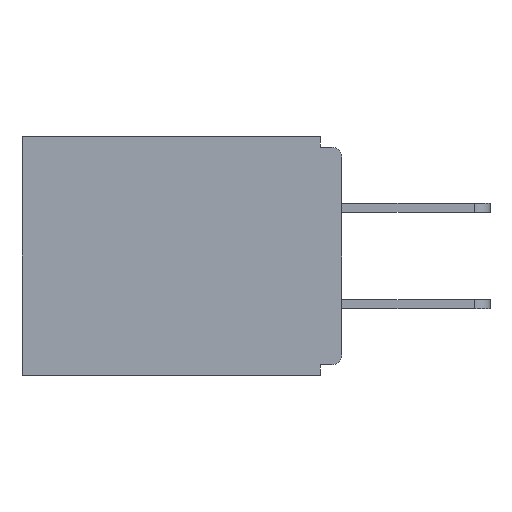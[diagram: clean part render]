
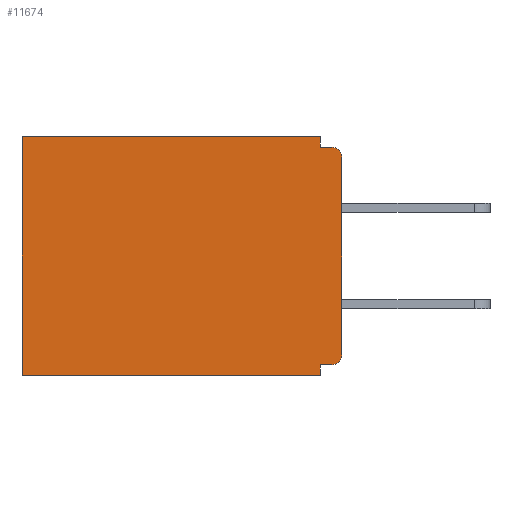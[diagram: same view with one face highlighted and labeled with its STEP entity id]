
A CAD part, left-side view. The second image highlights one B-rep face of the part: STEP entity #11674.
In plain terms, the highlighted planar face has unit normal (-1, 0, 0).
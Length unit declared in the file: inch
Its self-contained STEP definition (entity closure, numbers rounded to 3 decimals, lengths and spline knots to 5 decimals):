
#292 = CARTESIAN_POINT ( 'NONE',  ( 0.298, 0.46, 0. ) ) ;
#1501 = CARTESIAN_POINT ( 'NONE',  ( 0.298, 0.46, -0.343 ) ) ;
#1560 = EDGE_CURVE ( 'NONE', #3547, #20844, #1726, .T. ) ;
#1709 = ORIENTED_EDGE ( 'NONE', *, *, #22914, .T. ) ;
#1726 = LINE ( 'NONE', #8115, #23802 ) ;
#1898 = EDGE_CURVE ( 'NONE', #21449, #11627, #26825, .T. ) ;
#2125 = EDGE_CURVE ( 'NONE', #12334, #6554, #13022, .T. ) ;
#2686 = EDGE_CURVE ( 'NONE', #12334, #3741, #8973, .T. ) ;
#2949 = DIRECTION ( 'NONE',  ( -1., 0., 0. ) ) ;
#3547 = VERTEX_POINT ( 'NONE', #9557 ) ;
#3594 = VECTOR ( 'NONE', #25266, 39.37008 ) ;
#3741 = VERTEX_POINT ( 'NONE', #12720 ) ;
#3879 = CARTESIAN_POINT ( 'NONE',  ( 0.298, 0., -0.328 ) ) ;
#4318 = DIRECTION ( 'NONE',  ( 0., 0., -1. ) ) ;
#5423 = DIRECTION ( 'NONE',  ( 0., 0., -1. ) ) ;
#5982 = AXIS2_PLACEMENT_3D ( 'NONE', #6267, #6542, #8585 ) ;
#6267 = CARTESIAN_POINT ( 'NONE',  ( 0.298, 0., 0. ) ) ;
#6319 = VECTOR ( 'NONE', #26836, 39.37008 ) ;
#6383 = ORIENTED_EDGE ( 'NONE', *, *, #1898, .F. ) ;
#6542 = DIRECTION ( 'NONE',  ( 1., 0., 0. ) ) ;
#6554 = VERTEX_POINT ( 'NONE', #20681 ) ;
#6801 = EDGE_CURVE ( 'NONE', #20652, #20844, #18402, .T. ) ;
#6886 = VERTEX_POINT ( 'NONE', #8029 ) ;
#6926 = LINE ( 'NONE', #23289, #3594 ) ;
#7665 = VECTOR ( 'NONE', #14417, 39.37008 ) ;
#7675 = CARTESIAN_POINT ( 'NONE',  ( 0.298, 0.031, -0.015 ) ) ;
#7689 = CARTESIAN_POINT ( 'NONE',  ( 0.298, 0.031, -0.343 ) ) ;
#7788 = ORIENTED_EDGE ( 'NONE', *, *, #21807, .F. ) ;
#7866 = DIRECTION ( 'NONE',  ( 0., 0., -1. ) ) ;
#8029 = CARTESIAN_POINT ( 'NONE',  ( 0.298, 0.015, -0.328 ) ) ;
#8115 = CARTESIAN_POINT ( 'NONE',  ( 0.298, 0., -0.343 ) ) ;
#8320 = LINE ( 'NONE', #3879, #7665 ) ;
#8585 = DIRECTION ( 'NONE',  ( 0., 0., -1. ) ) ;
#8672 = PLANE ( 'NONE',  #5982 ) ;
#8973 = LINE ( 'NONE', #9765, #6319 ) ;
#9009 = CIRCLE ( 'NONE', #10840, 0.015 ) ;
#9113 = DIRECTION ( 'NONE',  ( 0., 1., 0. ) ) ;
#9505 = CARTESIAN_POINT ( 'NONE',  ( 0.298, 0.015, -0.313 ) ) ;
#9557 = CARTESIAN_POINT ( 'NONE',  ( 0.298, 0.031, -0.343 ) ) ;
#9765 = CARTESIAN_POINT ( 'NONE',  ( 0.298, 0., 0. ) ) ;
#10840 = AXIS2_PLACEMENT_3D ( 'NONE', #9505, #2949, #15634 ) ;
#11262 = VECTOR ( 'NONE', #9113, 39.37008 ) ;
#11627 = VERTEX_POINT ( 'NONE', #7675 ) ;
#11650 = DIRECTION ( 'NONE',  ( 0., 0., -1. ) ) ;
#11674 = ADVANCED_FACE ( 'NONE', ( #25546 ), #8672, .F. ) ;
#12334 = VERTEX_POINT ( 'NONE', #27277 ) ;
#12720 = CARTESIAN_POINT ( 'NONE',  ( 0.298, 0., -0.313 ) ) ;
#12812 = ORIENTED_EDGE ( 'NONE', *, *, #1560, .F. ) ;
#13022 = CIRCLE ( 'NONE', #13115, 0.015 ) ;
#13115 = AXIS2_PLACEMENT_3D ( 'NONE', #21330, #25677, #4318 ) ;
#13514 = EDGE_CURVE ( 'NONE', #6886, #3741, #9009, .T. ) ;
#13650 = EDGE_CURVE ( 'NONE', #6886, #24171, #8320, .T. ) ;
#14006 = ORIENTED_EDGE ( 'NONE', *, *, #13514, .T. ) ;
#14270 = LINE ( 'NONE', #7689, #20623 ) ;
#14417 = DIRECTION ( 'NONE',  ( 0., 1., 0. ) ) ;
#15634 = DIRECTION ( 'NONE',  ( 0., 0., -1. ) ) ;
#17066 = VECTOR ( 'NONE', #5423, 39.37008 ) ;
#17475 = CARTESIAN_POINT ( 'NONE',  ( 0.298, 0., 0. ) ) ;
#17626 = CARTESIAN_POINT ( 'NONE',  ( 0.298, 0.031, 0. ) ) ;
#18048 = CARTESIAN_POINT ( 'NONE',  ( 0.298, 0.031, -0.328 ) ) ;
#18402 = LINE ( 'NONE', #24947, #17066 ) ;
#19158 = ORIENTED_EDGE ( 'NONE', *, *, #2125, .T. ) ;
#20623 = VECTOR ( 'NONE', #7866, 39.37008 ) ;
#20652 = VERTEX_POINT ( 'NONE', #292 ) ;
#20681 = CARTESIAN_POINT ( 'NONE',  ( 0.298, 0.015, -0.015 ) ) ;
#20844 = VERTEX_POINT ( 'NONE', #1501 ) ;
#21330 = CARTESIAN_POINT ( 'NONE',  ( 0.298, 0.015, -0.03 ) ) ;
#21449 = VERTEX_POINT ( 'NONE', #17626 ) ;
#21807 = EDGE_CURVE ( 'NONE', #11627, #6554, #6926, .T. ) ;
#22551 = EDGE_CURVE ( 'NONE', #24171, #3547, #14270, .T. ) ;
#22914 = EDGE_CURVE ( 'NONE', #21449, #20652, #27720, .T. ) ;
#23289 = CARTESIAN_POINT ( 'NONE',  ( 0.298, 0., -0.015 ) ) ;
#23802 = VECTOR ( 'NONE', #25527, 39.37008 ) ;
#24171 = VERTEX_POINT ( 'NONE', #18048 ) ;
#24198 = ORIENTED_EDGE ( 'NONE', *, *, #6801, .T. ) ;
#24474 = CARTESIAN_POINT ( 'NONE',  ( 0.298, 0.031, -0.343 ) ) ;
#24766 = VECTOR ( 'NONE', #11650, 39.37008 ) ;
#24873 = ORIENTED_EDGE ( 'NONE', *, *, #2686, .F. ) ;
#24947 = CARTESIAN_POINT ( 'NONE',  ( 0.298, 0.46, 0. ) ) ;
#25041 = ORIENTED_EDGE ( 'NONE', *, *, #22551, .F. ) ;
#25266 = DIRECTION ( 'NONE',  ( 0., -1., 0. ) ) ;
#25527 = DIRECTION ( 'NONE',  ( 0., 1., 0. ) ) ;
#25546 = FACE_OUTER_BOUND ( 'NONE', #27232, .T. ) ;
#25677 = DIRECTION ( 'NONE',  ( -1., 0., 0. ) ) ;
#26377 = ORIENTED_EDGE ( 'NONE', *, *, #13650, .F. ) ;
#26825 = LINE ( 'NONE', #24474, #24766 ) ;
#26836 = DIRECTION ( 'NONE',  ( 0., 0., -1. ) ) ;
#27232 = EDGE_LOOP ( 'NONE', ( #19158, #7788, #6383, #1709, #24198, #12812, #25041, #26377, #14006, #24873 ) ) ;
#27277 = CARTESIAN_POINT ( 'NONE',  ( 0.298, 0., -0.03 ) ) ;
#27720 = LINE ( 'NONE', #17475, #11262 ) ;
